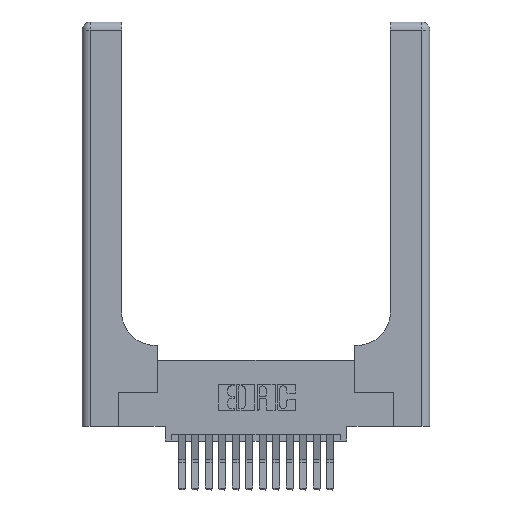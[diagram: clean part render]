
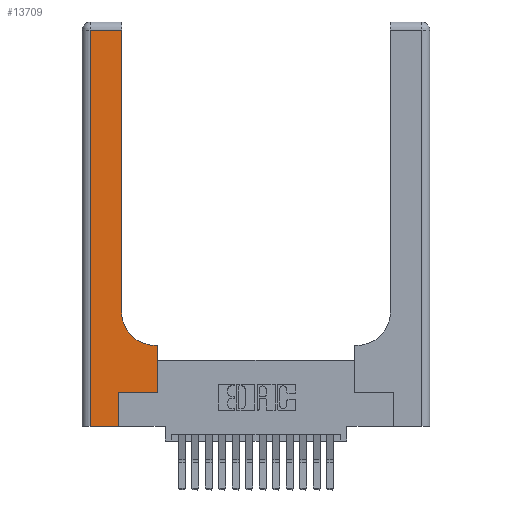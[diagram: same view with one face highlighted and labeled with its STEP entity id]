
A CAD part, top view. The second image highlights one B-rep face of the part: STEP entity #13709.
In plain terms, the highlighted planar face has unit normal (0, 0, 1).
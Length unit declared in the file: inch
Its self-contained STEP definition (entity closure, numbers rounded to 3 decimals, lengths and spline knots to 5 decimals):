
#118 = EDGE_CURVE ( 'NONE', #11961, #14559, #9371, .T. ) ;
#483 = ORIENTED_EDGE ( 'NONE', *, *, #16627, .T. ) ;
#1057 = LINE ( 'NONE', #8353, #12256 ) ;
#1232 = EDGE_CURVE ( 'NONE', #10248, #12745, #17999, .T. ) ;
#1679 = EDGE_CURVE ( 'NONE', #14346, #2293, #15081, .T. ) ;
#1811 = CARTESIAN_POINT ( 'NONE',  ( 0., 2.94, 0.37 ) ) ;
#1851 = DIRECTION ( 'NONE',  ( -1., 0., 0. ) ) ;
#2293 = VERTEX_POINT ( 'NONE', #2926 ) ;
#2912 = EDGE_CURVE ( 'NONE', #2293, #11961, #11400, .T. ) ;
#2926 = CARTESIAN_POINT ( 'NONE',  ( 0.2915, 2.94, 0.37 ) ) ;
#3174 = DIRECTION ( 'NONE',  ( 0., 0., -1. ) ) ;
#3384 = AXIS2_PLACEMENT_3D ( 'NONE', #11946, #3174, #13425 ) ;
#3779 = DIRECTION ( 'NONE',  ( 0., 1., 0. ) ) ;
#3878 = VECTOR ( 'NONE', #16342, 39.37008 ) ;
#4055 = VECTOR ( 'NONE', #1851, 39.37008 ) ;
#5053 = EDGE_CURVE ( 'NONE', #11001, #10248, #1057, .T. ) ;
#5179 = CARTESIAN_POINT ( 'NONE',  ( 0.269, 0.25, 0.37 ) ) ;
#5326 = CARTESIAN_POINT ( 'NONE',  ( 0.06, 2.94, 0.37 ) ) ;
#5492 = EDGE_LOOP ( 'NONE', ( #17169, #7473, #10494, #18139, #8198, #17577, #16393, #483, #8957 ) ) ;
#5845 = CARTESIAN_POINT ( 'NONE',  ( 0., 0., 0.37 ) ) ;
#6259 = DIRECTION ( 'NONE',  ( -1., 0., 0. ) ) ;
#6293 = AXIS2_PLACEMENT_3D ( 'NONE', #12489, #6664, #16863 ) ;
#6370 = VECTOR ( 'NONE', #14039, 39.37008 ) ;
#6396 = VECTOR ( 'NONE', #6259, 39.37008 ) ;
#6664 = DIRECTION ( 'NONE',  ( 0., 0., -1. ) ) ;
#7197 = VERTEX_POINT ( 'NONE', #17125 ) ;
#7464 = EDGE_CURVE ( 'NONE', #12956, #14346, #8746, .T. ) ;
#7473 = ORIENTED_EDGE ( 'NONE', *, *, #2912, .T. ) ;
#8198 = ORIENTED_EDGE ( 'NONE', *, *, #10447, .T. ) ;
#8353 = CARTESIAN_POINT ( 'NONE',  ( 0.269, 0.25, 0.37 ) ) ;
#8467 = VECTOR ( 'NONE', #9176, 39.37008 ) ;
#8746 = CIRCLE ( 'NONE', #3384, 0.25 ) ;
#8957 = ORIENTED_EDGE ( 'NONE', *, *, #7464, .T. ) ;
#9176 = DIRECTION ( 'NONE',  ( 0., -1., 0. ) ) ;
#9371 = LINE ( 'NONE', #10753, #8467 ) ;
#9623 = CARTESIAN_POINT ( 'NONE',  ( 0.269, 0., 0.37 ) ) ;
#9845 = LINE ( 'NONE', #15013, #6396 ) ;
#10248 = VERTEX_POINT ( 'NONE', #10630 ) ;
#10447 = EDGE_CURVE ( 'NONE', #7197, #11001, #15505, .T. ) ;
#10494 = ORIENTED_EDGE ( 'NONE', *, *, #118, .T. ) ;
#10615 = FACE_OUTER_BOUND ( 'NONE', #5492, .T. ) ;
#10630 = CARTESIAN_POINT ( 'NONE',  ( 0.5585, 0.25, 0.37 ) ) ;
#10753 = CARTESIAN_POINT ( 'NONE',  ( 0.06, 3., 0.37 ) ) ;
#11001 = VERTEX_POINT ( 'NONE', #5179 ) ;
#11400 = LINE ( 'NONE', #1811, #4055 ) ;
#11446 = VECTOR ( 'NONE', #3779, 39.37008 ) ;
#11621 = EDGE_CURVE ( 'NONE', #14559, #7197, #16857, .T. ) ;
#11638 = CARTESIAN_POINT ( 'NONE',  ( 0.2915, 0.85, 0.37 ) ) ;
#11946 = CARTESIAN_POINT ( 'NONE',  ( 0.5415, 0.85, 0.37 ) ) ;
#11961 = VERTEX_POINT ( 'NONE', #5326 ) ;
#12256 = VECTOR ( 'NONE', #14235, 39.37008 ) ;
#12489 = CARTESIAN_POINT ( 'NONE',  ( 0., 3., 0.37 ) ) ;
#12745 = VERTEX_POINT ( 'NONE', #17467 ) ;
#12956 = VERTEX_POINT ( 'NONE', #13529 ) ;
#13193 = DIRECTION ( 'NONE',  ( 1., 0., 0. ) ) ;
#13425 = DIRECTION ( 'NONE',  ( 1., 0., 0. ) ) ;
#13529 = CARTESIAN_POINT ( 'NONE',  ( 0.5415, 0.6, 0.37 ) ) ;
#13605 = CARTESIAN_POINT ( 'NONE',  ( 0.06, 0., 0.37 ) ) ;
#13709 = ADVANCED_FACE ( 'NONE', ( #10615 ), #15405, .F. ) ;
#14039 = DIRECTION ( 'NONE',  ( 0., 1., 0. ) ) ;
#14235 = DIRECTION ( 'NONE',  ( 1., 0., 0. ) ) ;
#14346 = VERTEX_POINT ( 'NONE', #11638 ) ;
#14559 = VERTEX_POINT ( 'NONE', #13605 ) ;
#15013 = CARTESIAN_POINT ( 'NONE',  ( 0.2915, 0.6, 0.37 ) ) ;
#15081 = LINE ( 'NONE', #16410, #3878 ) ;
#15405 = PLANE ( 'NONE',  #6293 ) ;
#15505 = LINE ( 'NONE', #9623, #11446 ) ;
#16058 = CARTESIAN_POINT ( 'NONE',  ( 0.5585, 0.25, 0.37 ) ) ;
#16342 = DIRECTION ( 'NONE',  ( 0., 1., 0. ) ) ;
#16386 = VECTOR ( 'NONE', #13193, 39.37008 ) ;
#16393 = ORIENTED_EDGE ( 'NONE', *, *, #1232, .T. ) ;
#16410 = CARTESIAN_POINT ( 'NONE',  ( 0.2915, 3., 0.37 ) ) ;
#16627 = EDGE_CURVE ( 'NONE', #12745, #12956, #9845, .T. ) ;
#16857 = LINE ( 'NONE', #5845, #16386 ) ;
#16863 = DIRECTION ( 'NONE',  ( -1., 0., 0. ) ) ;
#17125 = CARTESIAN_POINT ( 'NONE',  ( 0.269, 0., 0.37 ) ) ;
#17169 = ORIENTED_EDGE ( 'NONE', *, *, #1679, .T. ) ;
#17467 = CARTESIAN_POINT ( 'NONE',  ( 0.5585, 0.6, 0.37 ) ) ;
#17577 = ORIENTED_EDGE ( 'NONE', *, *, #5053, .T. ) ;
#17999 = LINE ( 'NONE', #16058, #6370 ) ;
#18139 = ORIENTED_EDGE ( 'NONE', *, *, #11621, .T. ) ;
